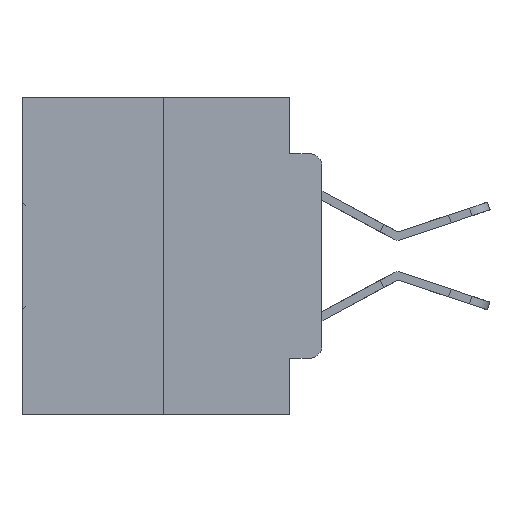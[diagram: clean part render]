
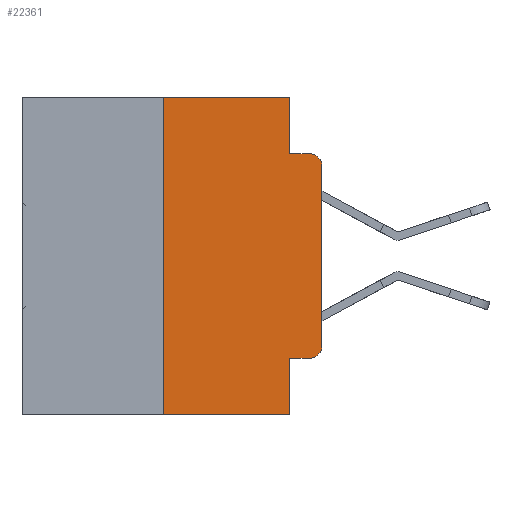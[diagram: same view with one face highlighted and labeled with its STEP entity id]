
A CAD part, left-side view. The second image highlights one B-rep face of the part: STEP entity #22361.
In plain terms, the highlighted planar face has unit normal (-1, 0, 0).
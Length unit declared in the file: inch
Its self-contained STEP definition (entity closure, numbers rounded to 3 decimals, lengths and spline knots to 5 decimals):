
#184 = DIRECTION ( 'NONE',  ( 0., 0., -1. ) ) ;
#328 = AXIS2_PLACEMENT_3D ( 'NONE', #30534, #13186, #22951 ) ;
#491 = DIRECTION ( 'NONE',  ( 0., -1., 0. ) ) ;
#1037 = AXIS2_PLACEMENT_3D ( 'NONE', #24890, #22701, #184 ) ;
#1263 = VECTOR ( 'NONE', #491, 39.37008 ) ;
#1434 = ORIENTED_EDGE ( 'NONE', *, *, #32389, .F. ) ;
#1690 = LINE ( 'NONE', #28616, #2060 ) ;
#1704 = EDGE_CURVE ( 'NONE', #20802, #9257, #5247, .T. ) ;
#2036 = VERTEX_POINT ( 'NONE', #22501 ) ;
#2060 = VECTOR ( 'NONE', #26312, 39.37008 ) ;
#2125 = EDGE_CURVE ( 'NONE', #2036, #10545, #13481, .T. ) ;
#3005 = ORIENTED_EDGE ( 'NONE', *, *, #9892, .T. ) ;
#3947 = CARTESIAN_POINT ( 'NONE',  ( 0., 0.25, 0. ) ) ;
#4042 = VERTEX_POINT ( 'NONE', #30604 ) ;
#4086 = VECTOR ( 'NONE', #14696, 39.37008 ) ;
#4267 = CARTESIAN_POINT ( 'NONE',  ( 0., 0.473, 0. ) ) ;
#4688 = EDGE_CURVE ( 'NONE', #16186, #10982, #31177, .T. ) ;
#4955 = CARTESIAN_POINT ( 'NONE',  ( 0., 0.02, -0.0885 ) ) ;
#5153 = DIRECTION ( 'NONE',  ( 0., 0., -1. ) ) ;
#5247 = LINE ( 'NONE', #19981, #4086 ) ;
#5388 = PLANE ( 'NONE',  #328 ) ;
#6661 = DIRECTION ( 'NONE',  ( 0., -1., 0. ) ) ;
#6728 = ORIENTED_EDGE ( 'NONE', *, *, #25433, .F. ) ;
#6733 = ORIENTED_EDGE ( 'NONE', *, *, #7654, .T. ) ;
#7654 = EDGE_CURVE ( 'NONE', #10982, #4042, #9317, .T. ) ;
#7942 = CARTESIAN_POINT ( 'NONE',  ( 0., 0.473, -0.5 ) ) ;
#8844 = CARTESIAN_POINT ( 'NONE',  ( 0., 0.051, -0.4115 ) ) ;
#9257 = VERTEX_POINT ( 'NONE', #4955 ) ;
#9317 = CIRCLE ( 'NONE', #1037, 0.02 ) ;
#9419 = DIRECTION ( 'NONE',  ( 0., 0., 1. ) ) ;
#9530 = CARTESIAN_POINT ( 'NONE',  ( 0., 0.25, 0. ) ) ;
#9636 = DIRECTION ( 'NONE',  ( 0., 0., 1. ) ) ;
#9892 = EDGE_CURVE ( 'NONE', #12644, #9257, #10063, .T. ) ;
#10030 = CARTESIAN_POINT ( 'NONE',  ( 0., 0.02, -0.4115 ) ) ;
#10063 = CIRCLE ( 'NONE', #10129, 0.02 ) ;
#10129 = AXIS2_PLACEMENT_3D ( 'NONE', #27281, #22595, #5153 ) ;
#10545 = VERTEX_POINT ( 'NONE', #23855 ) ;
#10982 = VERTEX_POINT ( 'NONE', #10030 ) ;
#12067 = VECTOR ( 'NONE', #29051, 39.37008 ) ;
#12327 = ORIENTED_EDGE ( 'NONE', *, *, #4688, .T. ) ;
#12644 = VERTEX_POINT ( 'NONE', #26085 ) ;
#13054 = EDGE_LOOP ( 'NONE', ( #24543, #3005, #21522, #25000, #1434, #15542, #27376, #6728, #12327, #6733 ) ) ;
#13186 = DIRECTION ( 'NONE',  ( 1., 0., 0. ) ) ;
#13481 = LINE ( 'NONE', #7942, #1263 ) ;
#13862 = VECTOR ( 'NONE', #6661, 39.37008 ) ;
#14696 = DIRECTION ( 'NONE',  ( 0., -1., 0. ) ) ;
#15542 = ORIENTED_EDGE ( 'NONE', *, *, #27411, .F. ) ;
#16186 = VERTEX_POINT ( 'NONE', #28488 ) ;
#16555 = CARTESIAN_POINT ( 'NONE',  ( 0., 0.051, 0. ) ) ;
#17264 = FACE_OUTER_BOUND ( 'NONE', #13054, .T. ) ;
#17795 = LINE ( 'NONE', #16555, #23682 ) ;
#19423 = DIRECTION ( 'NONE',  ( 0., 0., -1. ) ) ;
#19860 = CARTESIAN_POINT ( 'NONE',  ( 0., 0., 0. ) ) ;
#19981 = CARTESIAN_POINT ( 'NONE',  ( 0., 0.051, -0.0885 ) ) ;
#20802 = VERTEX_POINT ( 'NONE', #27070 ) ;
#21522 = ORIENTED_EDGE ( 'NONE', *, *, #1704, .F. ) ;
#22361 = ADVANCED_FACE ( 'NONE', ( #17264 ), #5388, .F. ) ;
#22501 = CARTESIAN_POINT ( 'NONE',  ( 0., 0.25, -0.5 ) ) ;
#22595 = DIRECTION ( 'NONE',  ( -1., 0., 0. ) ) ;
#22648 = LINE ( 'NONE', #4267, #12067 ) ;
#22701 = DIRECTION ( 'NONE',  ( -1., 0., 0. ) ) ;
#22951 = DIRECTION ( 'NONE',  ( 0., 0., -1. ) ) ;
#23682 = VECTOR ( 'NONE', #19423, 39.37008 ) ;
#23855 = CARTESIAN_POINT ( 'NONE',  ( 0., 0.051, -0.5 ) ) ;
#24543 = ORIENTED_EDGE ( 'NONE', *, *, #27526, .T. ) ;
#24890 = CARTESIAN_POINT ( 'NONE',  ( 0., 0.02, -0.3915 ) ) ;
#25000 = ORIENTED_EDGE ( 'NONE', *, *, #25306, .F. ) ;
#25306 = EDGE_CURVE ( 'NONE', #28007, #20802, #1690, .T. ) ;
#25433 = EDGE_CURVE ( 'NONE', #16186, #10545, #17795, .T. ) ;
#26085 = CARTESIAN_POINT ( 'NONE',  ( 0., 0., -0.1085 ) ) ;
#26311 = LINE ( 'NONE', #9530, #27876 ) ;
#26312 = DIRECTION ( 'NONE',  ( 0., 0., -1. ) ) ;
#26605 = CARTESIAN_POINT ( 'NONE',  ( 0., 0.051, 0. ) ) ;
#26719 = LINE ( 'NONE', #19860, #30290 ) ;
#27070 = CARTESIAN_POINT ( 'NONE',  ( 0., 0.051, -0.0885 ) ) ;
#27278 = VERTEX_POINT ( 'NONE', #3947 ) ;
#27281 = CARTESIAN_POINT ( 'NONE',  ( 0., 0.02, -0.1085 ) ) ;
#27376 = ORIENTED_EDGE ( 'NONE', *, *, #2125, .T. ) ;
#27411 = EDGE_CURVE ( 'NONE', #2036, #27278, #26311, .T. ) ;
#27526 = EDGE_CURVE ( 'NONE', #4042, #12644, #26719, .T. ) ;
#27876 = VECTOR ( 'NONE', #9419, 39.37008 ) ;
#28007 = VERTEX_POINT ( 'NONE', #26605 ) ;
#28488 = CARTESIAN_POINT ( 'NONE',  ( 0., 0.051, -0.4115 ) ) ;
#28616 = CARTESIAN_POINT ( 'NONE',  ( 0., 0.051, 0. ) ) ;
#29051 = DIRECTION ( 'NONE',  ( 0., -1., 0. ) ) ;
#30290 = VECTOR ( 'NONE', #9636, 39.37008 ) ;
#30534 = CARTESIAN_POINT ( 'NONE',  ( 0., 0.473, 0. ) ) ;
#30604 = CARTESIAN_POINT ( 'NONE',  ( 0., 0., -0.3915 ) ) ;
#31177 = LINE ( 'NONE', #8844, #13862 ) ;
#32389 = EDGE_CURVE ( 'NONE', #27278, #28007, #22648, .T. ) ;
